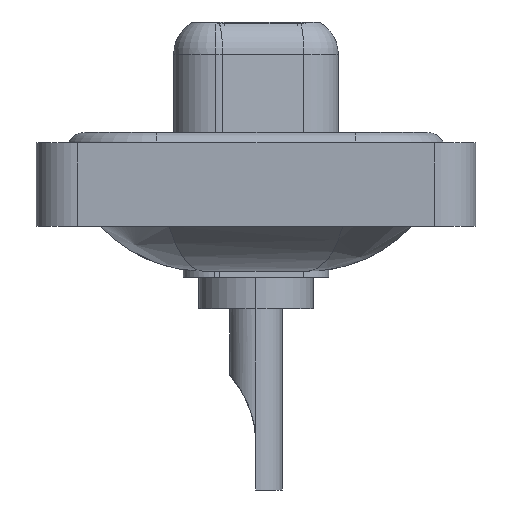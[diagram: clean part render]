
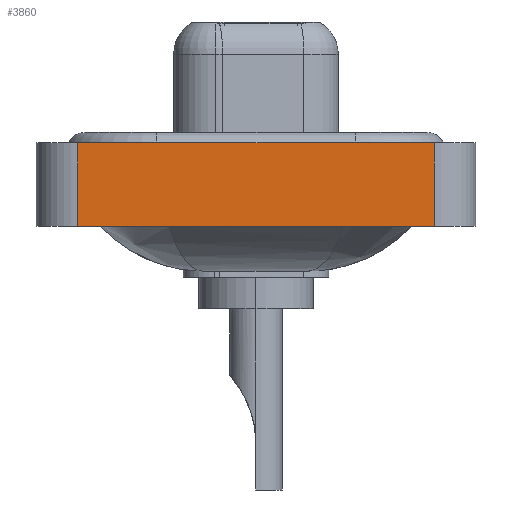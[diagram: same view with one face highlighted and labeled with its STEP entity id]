
A CAD part, left-side view. The second image highlights one B-rep face of the part: STEP entity #3860.
In plain terms, the highlighted planar face has unit normal (-1, 0, 0).
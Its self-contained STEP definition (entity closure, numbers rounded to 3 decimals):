
#68 = PLANE ( 'NONE',  #13707 ) ;
#186 = LINE ( 'NONE', #5271, #3935 ) ;
#937 = EDGE_CURVE ( 'NONE', #15548, #11515, #13805, .T. ) ;
#1288 = DIRECTION ( 'NONE',  ( 0., -1., 0. ) ) ;
#1445 = EDGE_CURVE ( 'NONE', #11515, #12353, #6242, .T. ) ;
#2716 = VECTOR ( 'NONE', #1288, 1000. ) ;
#3852 = DIRECTION ( 'NONE',  ( 0., 0., 1. ) ) ;
#3860 = ADVANCED_FACE ( 'NONE', ( #6383 ), #68, .T. ) ;
#3935 = VECTOR ( 'NONE', #3852, 1000. ) ;
#4254 = CARTESIAN_POINT ( 'NONE',  ( -7.3, -8.55, 0.4 ) ) ;
#4463 = CARTESIAN_POINT ( 'NONE',  ( -7.3, -8.55, -3.6 ) ) ;
#4772 = VERTEX_POINT ( 'NONE', #10539 ) ;
#5091 = EDGE_LOOP ( 'NONE', ( #15232, #5656, #7919, #8831 ) ) ;
#5271 = CARTESIAN_POINT ( 'NONE',  ( -7.3, 8.55, -3.6 ) ) ;
#5656 = ORIENTED_EDGE ( 'NONE', *, *, #6162, .F. ) ;
#6162 = EDGE_CURVE ( 'NONE', #4772, #12353, #15593, .T. ) ;
#6242 = LINE ( 'NONE', #13698, #10537 ) ;
#6383 = FACE_OUTER_BOUND ( 'NONE', #5091, .T. ) ;
#7063 = VECTOR ( 'NONE', #9229, 1000. ) ;
#7919 = ORIENTED_EDGE ( 'NONE', *, *, #7932, .F. ) ;
#7932 = EDGE_CURVE ( 'NONE', #15548, #4772, #186, .T. ) ;
#8581 = CARTESIAN_POINT ( 'NONE',  ( -7.3, -8.55, 0.4 ) ) ;
#8831 = ORIENTED_EDGE ( 'NONE', *, *, #937, .T. ) ;
#9229 = DIRECTION ( 'NONE',  ( 0., -1., 0. ) ) ;
#9865 = CARTESIAN_POINT ( 'NONE',  ( -7.3, -8.55, -3.6 ) ) ;
#10080 = CARTESIAN_POINT ( 'NONE',  ( -7.3, -8.55, -3.6 ) ) ;
#10537 = VECTOR ( 'NONE', #13607, 1000. ) ;
#10539 = CARTESIAN_POINT ( 'NONE',  ( -7.3, 8.55, 0.4 ) ) ;
#11515 = VERTEX_POINT ( 'NONE', #9865 ) ;
#11921 = DIRECTION ( 'NONE',  ( -1., 0., 0. ) ) ;
#12353 = VERTEX_POINT ( 'NONE', #8581 ) ;
#13073 = DIRECTION ( 'NONE',  ( 0., 0., 1. ) ) ;
#13607 = DIRECTION ( 'NONE',  ( 0., 0., 1. ) ) ;
#13698 = CARTESIAN_POINT ( 'NONE',  ( -7.3, -8.55, -3.6 ) ) ;
#13707 = AXIS2_PLACEMENT_3D ( 'NONE', #4463, #11921, #13073 ) ;
#13805 = LINE ( 'NONE', #10080, #2716 ) ;
#14930 = CARTESIAN_POINT ( 'NONE',  ( -7.3, 8.55, -3.6 ) ) ;
#15232 = ORIENTED_EDGE ( 'NONE', *, *, #1445, .T. ) ;
#15548 = VERTEX_POINT ( 'NONE', #14930 ) ;
#15593 = LINE ( 'NONE', #4254, #7063 ) ;
